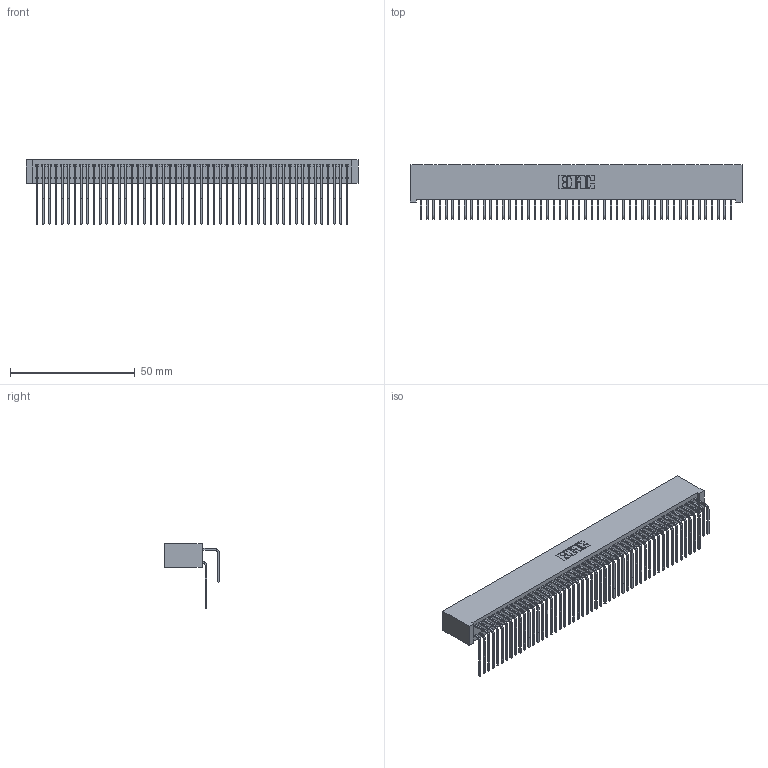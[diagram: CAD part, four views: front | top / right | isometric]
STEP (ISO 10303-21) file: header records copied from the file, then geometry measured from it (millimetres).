
FILE_DESCRIPTION (( 'STEP AP203' ), '1' );
FILE_NAME ('342-100-558-201.STEP', '2019-10-04T17:50:45', ( '' ), ( '' ), 'SwSTEP 2.0', 'SolidWorks 2016', '' );
FILE_SCHEMA (( 'CONFIG_CONTROL_DESIGN' ));
Length unit declared in the file: inch
Products named in the file (4): 345-292-001_558 559 Tail - 1; 345-292-001_558 Tail - 2; 342-100-558-201; 342 Part_Lugless
Assembly tree (101 placements, depth 2):
  342-100-558-201
    342 Part_Lugless
    345-292-001_558 559 Tail - 1  x50
    345-292-001_558 Tail - 2  x50
Bounding box: 133.25 x 21.91 x 25.78 mm (x, y, z)
Volume: 13026.6 mm3; surface area: 24457 mm2
Topology: 101 solids, 101 shells, 5502 faces, 16375 edges, 10782 vertices
Faces by surface type: plane 3862, cylinder 1640
Entity records: 32507 total; most frequent: CARTESIAN_POINT 5425, ORIENTED_EDGE 5310, DIRECTION 4595, EDGE_CURVE 2655, VECTOR 2495, LINE 2495, VERTEX_POINT 1766, AXIS2_PLACEMENT_3D 1050
